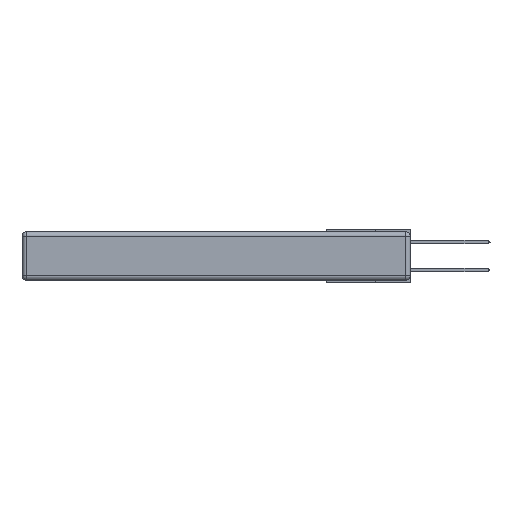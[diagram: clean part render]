
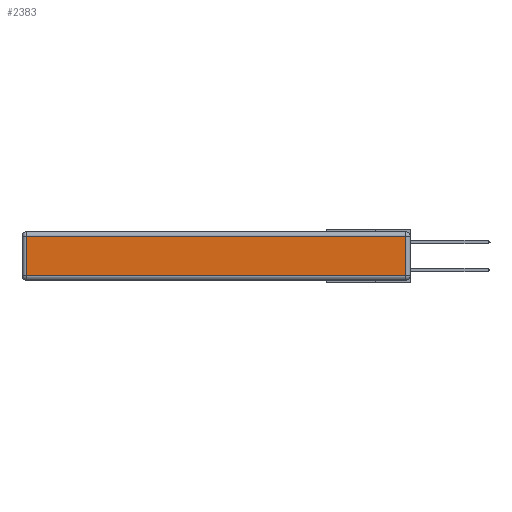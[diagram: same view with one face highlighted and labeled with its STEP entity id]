
A CAD part, left-side view. The second image highlights one B-rep face of the part: STEP entity #2383.
In plain terms, the highlighted planar face has unit normal (-1, 0, 0).
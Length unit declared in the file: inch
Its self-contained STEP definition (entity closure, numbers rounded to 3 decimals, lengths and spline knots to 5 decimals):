
#312 = EDGE_CURVE ( 'NONE', #16036, #4585, #8864, .T. ) ;
#399 = LINE ( 'NONE', #6218, #610 ) ;
#442 = EDGE_CURVE ( 'NONE', #14276, #16036, #986, .T. ) ;
#610 = VECTOR ( 'NONE', #3319, 39.37008 ) ;
#787 = VECTOR ( 'NONE', #14750, 39.37008 ) ;
#986 = LINE ( 'NONE', #18208, #16760 ) ;
#2103 = CARTESIAN_POINT ( 'NONE',  ( 0., 0.03, -0.313 ) ) ;
#2383 = ADVANCED_FACE ( 'NONE', ( #15058 ), #10544, .T. ) ;
#3319 = DIRECTION ( 'NONE',  ( 0., -1., 0. ) ) ;
#3975 = LINE ( 'NONE', #4397, #18803 ) ;
#4397 = CARTESIAN_POINT ( 'NONE',  ( 0., 2.72, -0.343 ) ) ;
#4585 = VERTEX_POINT ( 'NONE', #6865 ) ;
#6187 = CARTESIAN_POINT ( 'NONE',  ( 0., 0., -0.343 ) ) ;
#6218 = CARTESIAN_POINT ( 'NONE',  ( 0., 0., -0.313 ) ) ;
#6865 = CARTESIAN_POINT ( 'NONE',  ( 0., 2.72, -0.03 ) ) ;
#7685 = ORIENTED_EDGE ( 'NONE', *, *, #442, .T. ) ;
#8864 = LINE ( 'NONE', #14551, #787 ) ;
#8890 = EDGE_CURVE ( 'NONE', #4585, #13983, #3975, .T. ) ;
#8992 = EDGE_LOOP ( 'NONE', ( #18631, #7685, #13463, #12633 ) ) ;
#10544 = PLANE ( 'NONE',  #13881 ) ;
#12250 = CARTESIAN_POINT ( 'NONE',  ( 0., 2.72, -0.313 ) ) ;
#12633 = ORIENTED_EDGE ( 'NONE', *, *, #8890, .T. ) ;
#13295 = CARTESIAN_POINT ( 'NONE',  ( 0., 0.03, -0.03 ) ) ;
#13463 = ORIENTED_EDGE ( 'NONE', *, *, #312, .T. ) ;
#13881 = AXIS2_PLACEMENT_3D ( 'NONE', #6187, #16300, #16554 ) ;
#13983 = VERTEX_POINT ( 'NONE', #12250 ) ;
#14276 = VERTEX_POINT ( 'NONE', #2103 ) ;
#14551 = CARTESIAN_POINT ( 'NONE',  ( 0., 2.75, -0.03 ) ) ;
#14670 = DIRECTION ( 'NONE',  ( 0., 0., -1. ) ) ;
#14750 = DIRECTION ( 'NONE',  ( 0., 1., 0. ) ) ;
#15058 = FACE_OUTER_BOUND ( 'NONE', #8992, .T. ) ;
#15548 = DIRECTION ( 'NONE',  ( 0., 0., 1. ) ) ;
#15561 = EDGE_CURVE ( 'NONE', #13983, #14276, #399, .T. ) ;
#16036 = VERTEX_POINT ( 'NONE', #13295 ) ;
#16300 = DIRECTION ( 'NONE',  ( -1., 0., 0. ) ) ;
#16554 = DIRECTION ( 'NONE',  ( 0., 0., 1. ) ) ;
#16760 = VECTOR ( 'NONE', #15548, 39.37008 ) ;
#18208 = CARTESIAN_POINT ( 'NONE',  ( 0., 0.03, -0.343 ) ) ;
#18631 = ORIENTED_EDGE ( 'NONE', *, *, #15561, .T. ) ;
#18803 = VECTOR ( 'NONE', #14670, 39.37008 ) ;
